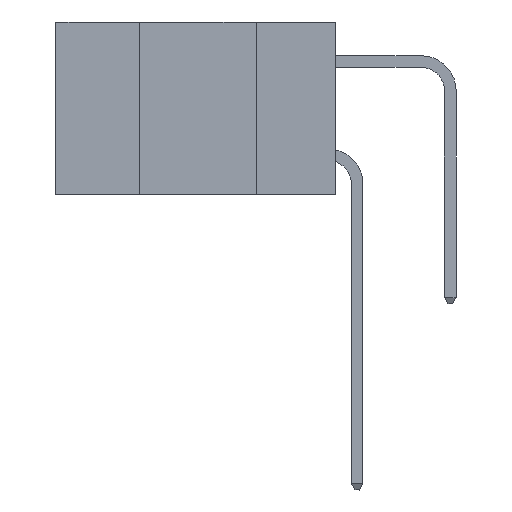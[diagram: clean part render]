
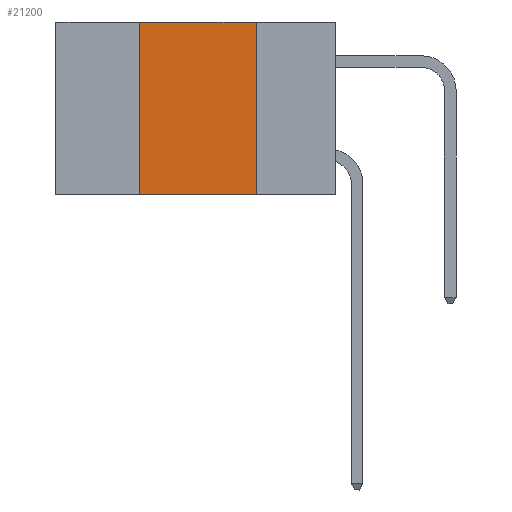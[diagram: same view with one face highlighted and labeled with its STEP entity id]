
A CAD part, left-side view. The second image highlights one B-rep face of the part: STEP entity #21200.
In plain terms, the highlighted planar face has unit normal (-1, 0, 0).
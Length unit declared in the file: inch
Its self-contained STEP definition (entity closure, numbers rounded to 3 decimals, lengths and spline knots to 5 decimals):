
#25 = AXIS2_PLACEMENT_3D ( 'NONE', #12304, #3755, #593 ) ;
#44 = VECTOR ( 'NONE', #5739, 39.37008 ) ;
#98 = EDGE_CURVE ( 'NONE', #12302, #15644, #4728, .T. ) ;
#551 = LINE ( 'NONE', #10689, #44 ) ;
#593 = DIRECTION ( 'NONE',  ( 0., 0., -1. ) ) ;
#1273 = VERTEX_POINT ( 'NONE', #1532 ) ;
#1532 = CARTESIAN_POINT ( 'NONE',  ( 0., 0.42, -0.37 ) ) ;
#2477 = EDGE_LOOP ( 'NONE', ( #11107, #4392, #20319, #17446 ) ) ;
#3536 = FACE_OUTER_BOUND ( 'NONE', #2477, .T. ) ;
#3755 = DIRECTION ( 'NONE',  ( 1., 0., 0. ) ) ;
#4392 = ORIENTED_EDGE ( 'NONE', *, *, #98, .F. ) ;
#4654 = EDGE_CURVE ( 'NONE', #15644, #9535, #4791, .T. ) ;
#4728 = LINE ( 'NONE', #10002, #16257 ) ;
#4791 = LINE ( 'NONE', #11984, #20589 ) ;
#5338 = PLANE ( 'NONE',  #25 ) ;
#5739 = DIRECTION ( 'NONE',  ( 0., -1., 0. ) ) ;
#7225 = CARTESIAN_POINT ( 'NONE',  ( 0., 0.42, 0. ) ) ;
#8602 = DIRECTION ( 'NONE',  ( 0., 0., -1. ) ) ;
#9535 = VERTEX_POINT ( 'NONE', #13771 ) ;
#10002 = CARTESIAN_POINT ( 'NONE',  ( 0., 0.6, 0. ) ) ;
#10689 = CARTESIAN_POINT ( 'NONE',  ( 0., 0.6, -0.37 ) ) ;
#11107 = ORIENTED_EDGE ( 'NONE', *, *, #4654, .F. ) ;
#11168 = EDGE_CURVE ( 'NONE', #1273, #12302, #19225, .T. ) ;
#11984 = CARTESIAN_POINT ( 'NONE',  ( 0., 0.17, 0. ) ) ;
#12302 = VERTEX_POINT ( 'NONE', #21632 ) ;
#12304 = CARTESIAN_POINT ( 'NONE',  ( 0., 0.6, 0. ) ) ;
#13771 = CARTESIAN_POINT ( 'NONE',  ( 0., 0.17, -0.37 ) ) ;
#13796 = CARTESIAN_POINT ( 'NONE',  ( 0., 0.17, 0. ) ) ;
#15169 = DIRECTION ( 'NONE',  ( 0., -1., 0. ) ) ;
#15644 = VERTEX_POINT ( 'NONE', #13796 ) ;
#16257 = VECTOR ( 'NONE', #15169, 39.37008 ) ;
#17446 = ORIENTED_EDGE ( 'NONE', *, *, #21808, .T. ) ;
#18410 = VECTOR ( 'NONE', #20915, 39.37008 ) ;
#19225 = LINE ( 'NONE', #7225, #18410 ) ;
#20319 = ORIENTED_EDGE ( 'NONE', *, *, #11168, .F. ) ;
#20589 = VECTOR ( 'NONE', #8602, 39.37008 ) ;
#20915 = DIRECTION ( 'NONE',  ( 0., 0., 1. ) ) ;
#21200 = ADVANCED_FACE ( 'NONE', ( #3536 ), #5338, .F. ) ;
#21632 = CARTESIAN_POINT ( 'NONE',  ( 0., 0.42, 0. ) ) ;
#21808 = EDGE_CURVE ( 'NONE', #1273, #9535, #551, .T. ) ;
